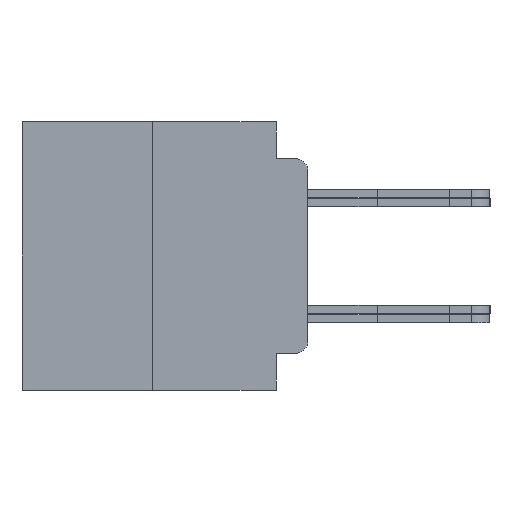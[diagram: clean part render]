
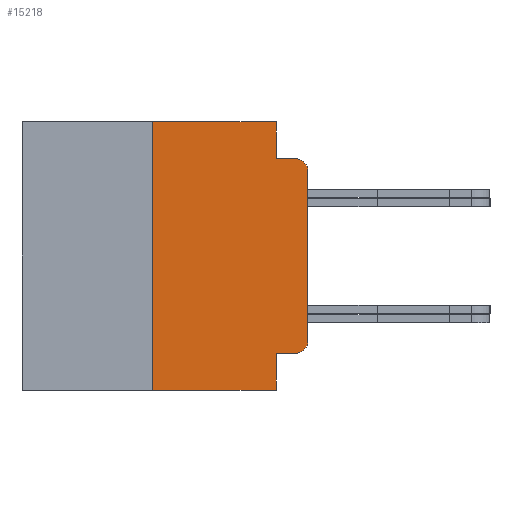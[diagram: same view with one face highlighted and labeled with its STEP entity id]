
A CAD part, left-side view. The second image highlights one B-rep face of the part: STEP entity #15218.
In plain terms, the highlighted planar face has unit normal (-1, 0, 0).
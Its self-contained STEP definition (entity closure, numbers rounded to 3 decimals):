
#1146 = CARTESIAN_POINT ( 'NONE',  ( -75.603, 11.684, 5.486 ) ) ;
#1154 = DIRECTION ( 'NONE',  ( 0., 0., 1. ) ) ;
#1417 = DIRECTION ( 'NONE',  ( 1., 0., 0. ) ) ;
#1747 = ORIENTED_EDGE ( 'NONE', *, *, #27236, .T. ) ;
#1837 = CARTESIAN_POINT ( 'NONE',  ( -75.603, 1.295, 0. ) ) ;
#1961 = VECTOR ( 'NONE', #5565, 1000. ) ;
#1979 = EDGE_CURVE ( 'NONE', #14167, #9143, #12982, .T. ) ;
#2055 = CARTESIAN_POINT ( 'NONE',  ( -75.603, 6.35, -5.486 ) ) ;
#2062 = EDGE_CURVE ( 'NONE', #12628, #14167, #13338, .T. ) ;
#3124 = EDGE_LOOP ( 'NONE', ( #17969, #21106, #1747, #18745, #24121, #21150, #10530, #12306, #17193, #26893 ) ) ;
#3228 = EDGE_CURVE ( 'NONE', #19421, #12294, #4638, .T. ) ;
#3384 = VERTEX_POINT ( 'NONE', #22556 ) ;
#4405 = LINE ( 'NONE', #2055, #8492 ) ;
#4522 = EDGE_CURVE ( 'NONE', #3384, #12294, #25340, .T. ) ;
#4638 = LINE ( 'NONE', #25107, #10488 ) ;
#5321 = DIRECTION ( 'NONE',  ( -1., 0., 0. ) ) ;
#5565 = DIRECTION ( 'NONE',  ( 0., -1., 0. ) ) ;
#6122 = DIRECTION ( 'NONE',  ( 0., 0., -1. ) ) ;
#6321 = CARTESIAN_POINT ( 'NONE',  ( -75.603, 1.295, -5.486 ) ) ;
#7789 = LINE ( 'NONE', #1146, #1961 ) ;
#7809 = EDGE_CURVE ( 'NONE', #3384, #21076, #15992, .T. ) ;
#8349 = CARTESIAN_POINT ( 'NONE',  ( -75.603, 0.508, 3.467 ) ) ;
#8440 = CARTESIAN_POINT ( 'NONE',  ( -75.603, 1.295, -3.975 ) ) ;
#8492 = VECTOR ( 'NONE', #17460, 1000. ) ;
#9143 = VERTEX_POINT ( 'NONE', #23658 ) ;
#10463 = VECTOR ( 'NONE', #17893, 1000. ) ;
#10488 = VECTOR ( 'NONE', #14277, 1000. ) ;
#10530 = ORIENTED_EDGE ( 'NONE', *, *, #25251, .F. ) ;
#10562 = CARTESIAN_POINT ( 'NONE',  ( -75.603, 11.684, 5.486 ) ) ;
#11628 = DIRECTION ( 'NONE',  ( -1., 0., 0. ) ) ;
#11875 = EDGE_CURVE ( 'NONE', #19421, #19969, #4405, .T. ) ;
#11945 = VECTOR ( 'NONE', #19366, 1000. ) ;
#12237 = LINE ( 'NONE', #16863, #23288 ) ;
#12294 = VERTEX_POINT ( 'NONE', #6321 ) ;
#12306 = ORIENTED_EDGE ( 'NONE', *, *, #11875, .F. ) ;
#12420 = CARTESIAN_POINT ( 'NONE',  ( -75.603, 1.295, 3.975 ) ) ;
#12628 = VERTEX_POINT ( 'NONE', #20733 ) ;
#12982 = LINE ( 'NONE', #12420, #17123 ) ;
#13338 = LINE ( 'NONE', #1837, #11945 ) ;
#13961 = AXIS2_PLACEMENT_3D ( 'NONE', #22677, #5321, #18628 ) ;
#14167 = VERTEX_POINT ( 'NONE', #23867 ) ;
#14277 = DIRECTION ( 'NONE',  ( 0., -1., 0. ) ) ;
#14571 = FACE_OUTER_BOUND ( 'NONE', #3124, .T. ) ;
#14819 = CARTESIAN_POINT ( 'NONE',  ( -75.603, 0.508, -3.975 ) ) ;
#15173 = CARTESIAN_POINT ( 'NONE',  ( -75.603, 6.35, 5.486 ) ) ;
#15218 = ADVANCED_FACE ( 'NONE', ( #14571 ), #19341, .F. ) ;
#15419 = CIRCLE ( 'NONE', #25634, 0.508 ) ;
#15568 = CARTESIAN_POINT ( 'NONE',  ( -75.603, 6.35, -5.486 ) ) ;
#15992 = LINE ( 'NONE', #8440, #20464 ) ;
#16863 = CARTESIAN_POINT ( 'NONE',  ( -75.603, 0., 5.486 ) ) ;
#17123 = VECTOR ( 'NONE', #25485, 1000. ) ;
#17193 = ORIENTED_EDGE ( 'NONE', *, *, #3228, .T. ) ;
#17460 = DIRECTION ( 'NONE',  ( 0., 0., 1. ) ) ;
#17893 = DIRECTION ( 'NONE',  ( 0., 0., -1. ) ) ;
#17969 = ORIENTED_EDGE ( 'NONE', *, *, #7809, .T. ) ;
#18287 = DIRECTION ( 'NONE',  ( 0., 0., -1. ) ) ;
#18628 = DIRECTION ( 'NONE',  ( 0., 0., -1. ) ) ;
#18745 = ORIENTED_EDGE ( 'NONE', *, *, #25582, .T. ) ;
#19341 = PLANE ( 'NONE',  #22288 ) ;
#19366 = DIRECTION ( 'NONE',  ( 0., 0., -1. ) ) ;
#19421 = VERTEX_POINT ( 'NONE', #15568 ) ;
#19691 = CARTESIAN_POINT ( 'NONE',  ( -75.603, 0., -3.467 ) ) ;
#19969 = VERTEX_POINT ( 'NONE', #15173 ) ;
#20464 = VECTOR ( 'NONE', #23814, 1000. ) ;
#20733 = CARTESIAN_POINT ( 'NONE',  ( -75.603, 1.295, 5.486 ) ) ;
#21076 = VERTEX_POINT ( 'NONE', #14819 ) ;
#21106 = ORIENTED_EDGE ( 'NONE', *, *, #24561, .T. ) ;
#21150 = ORIENTED_EDGE ( 'NONE', *, *, #2062, .F. ) ;
#22288 = AXIS2_PLACEMENT_3D ( 'NONE', #10562, #1417, #6122 ) ;
#22556 = CARTESIAN_POINT ( 'NONE',  ( -75.603, 1.295, -3.975 ) ) ;
#22677 = CARTESIAN_POINT ( 'NONE',  ( -75.603, 0.508, -3.467 ) ) ;
#23288 = VECTOR ( 'NONE', #1154, 1000. ) ;
#23658 = CARTESIAN_POINT ( 'NONE',  ( -75.603, 0.508, 3.975 ) ) ;
#23814 = DIRECTION ( 'NONE',  ( 0., -1., 0. ) ) ;
#23867 = CARTESIAN_POINT ( 'NONE',  ( -75.603, 1.295, 3.975 ) ) ;
#24121 = ORIENTED_EDGE ( 'NONE', *, *, #1979, .F. ) ;
#24127 = CIRCLE ( 'NONE', #13961, 0.508 ) ;
#24561 = EDGE_CURVE ( 'NONE', #21076, #26813, #24127, .T. ) ;
#24666 = CARTESIAN_POINT ( 'NONE',  ( -75.603, 1.295, 0. ) ) ;
#25107 = CARTESIAN_POINT ( 'NONE',  ( -75.603, 11.684, -5.486 ) ) ;
#25251 = EDGE_CURVE ( 'NONE', #19969, #12628, #7789, .T. ) ;
#25340 = LINE ( 'NONE', #24666, #10463 ) ;
#25485 = DIRECTION ( 'NONE',  ( 0., -1., 0. ) ) ;
#25582 = EDGE_CURVE ( 'NONE', #28344, #9143, #15419, .T. ) ;
#25634 = AXIS2_PLACEMENT_3D ( 'NONE', #8349, #11628, #18287 ) ;
#26813 = VERTEX_POINT ( 'NONE', #19691 ) ;
#26893 = ORIENTED_EDGE ( 'NONE', *, *, #4522, .F. ) ;
#26934 = CARTESIAN_POINT ( 'NONE',  ( -75.603, 0., 3.467 ) ) ;
#27236 = EDGE_CURVE ( 'NONE', #26813, #28344, #12237, .T. ) ;
#28344 = VERTEX_POINT ( 'NONE', #26934 ) ;
